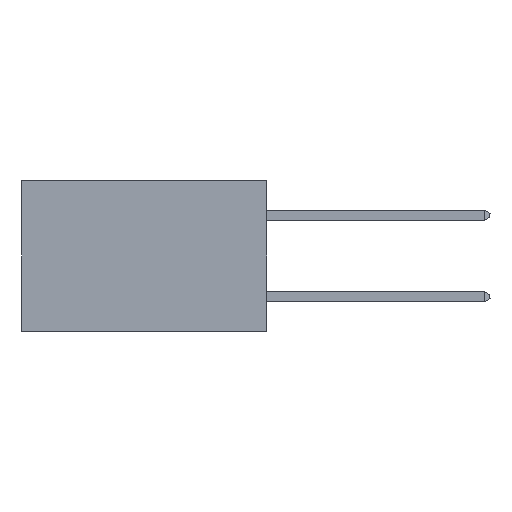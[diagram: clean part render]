
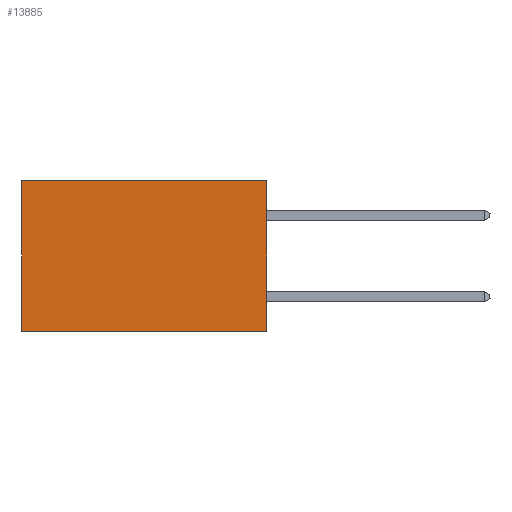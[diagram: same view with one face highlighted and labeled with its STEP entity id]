
A CAD part, left-side view. The second image highlights one B-rep face of the part: STEP entity #13885.
In plain terms, the highlighted planar face has unit normal (-1, 0, 0).
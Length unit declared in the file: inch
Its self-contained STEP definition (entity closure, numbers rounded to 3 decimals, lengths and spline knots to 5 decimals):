
#341 = ORIENTED_EDGE ( 'NONE', *, *, #1765, .T. ) ;
#1135 = CARTESIAN_POINT ( 'NONE',  ( 0.2875, 0., 0. ) ) ;
#1177 = LINE ( 'NONE', #5328, #5327 ) ;
#1494 = VECTOR ( 'NONE', #4915, 39.37008 ) ;
#1643 = CARTESIAN_POINT ( 'NONE',  ( 0.2875, 0., 0. ) ) ;
#1765 = EDGE_CURVE ( 'NONE', #2931, #14576, #2944, .T. ) ;
#2632 = LINE ( 'NONE', #3739, #17344 ) ;
#2931 = VERTEX_POINT ( 'NONE', #1643 ) ;
#2944 = LINE ( 'NONE', #9550, #1494 ) ;
#3739 = CARTESIAN_POINT ( 'NONE',  ( 0.2875, 0., 0. ) ) ;
#4915 = DIRECTION ( 'NONE',  ( 0., 1., 0. ) ) ;
#4953 = CARTESIAN_POINT ( 'NONE',  ( 0.2875, 0.6, 0. ) ) ;
#5327 = VECTOR ( 'NONE', #19349, 39.37008 ) ;
#5328 = CARTESIAN_POINT ( 'NONE',  ( 0.2875, 0., -0.37 ) ) ;
#5483 = LINE ( 'NONE', #7289, #16790 ) ;
#7251 = VERTEX_POINT ( 'NONE', #15155 ) ;
#7289 = CARTESIAN_POINT ( 'NONE',  ( 0.2875, 0.6, 0. ) ) ;
#7855 = ORIENTED_EDGE ( 'NONE', *, *, #9659, .F. ) ;
#8216 = AXIS2_PLACEMENT_3D ( 'NONE', #1135, #18287, #11937 ) ;
#8925 = ORIENTED_EDGE ( 'NONE', *, *, #16748, .F. ) ;
#9550 = CARTESIAN_POINT ( 'NONE',  ( 0.2875, 0., 0. ) ) ;
#9659 = EDGE_CURVE ( 'NONE', #7251, #12615, #1177, .T. ) ;
#10558 = PLANE ( 'NONE',  #8216 ) ;
#11338 = EDGE_CURVE ( 'NONE', #14576, #12615, #5483, .T. ) ;
#11937 = DIRECTION ( 'NONE',  ( 0., 0., -1. ) ) ;
#11959 = ORIENTED_EDGE ( 'NONE', *, *, #11338, .T. ) ;
#12615 = VERTEX_POINT ( 'NONE', #16742 ) ;
#13779 = DIRECTION ( 'NONE',  ( 0., 0., -1. ) ) ;
#13885 = ADVANCED_FACE ( 'NONE', ( #17242 ), #10558, .F. ) ;
#14576 = VERTEX_POINT ( 'NONE', #4953 ) ;
#14744 = EDGE_LOOP ( 'NONE', ( #11959, #7855, #8925, #341 ) ) ;
#15155 = CARTESIAN_POINT ( 'NONE',  ( 0.2875, 0., -0.37 ) ) ;
#16742 = CARTESIAN_POINT ( 'NONE',  ( 0.2875, 0.6, -0.37 ) ) ;
#16748 = EDGE_CURVE ( 'NONE', #2931, #7251, #2632, .T. ) ;
#16790 = VECTOR ( 'NONE', #13779, 39.37008 ) ;
#17242 = FACE_OUTER_BOUND ( 'NONE', #14744, .T. ) ;
#17344 = VECTOR ( 'NONE', #19675, 39.37008 ) ;
#18287 = DIRECTION ( 'NONE',  ( 1., 0., 0. ) ) ;
#19349 = DIRECTION ( 'NONE',  ( 0., 1., 0. ) ) ;
#19675 = DIRECTION ( 'NONE',  ( 0., 0., -1. ) ) ;
